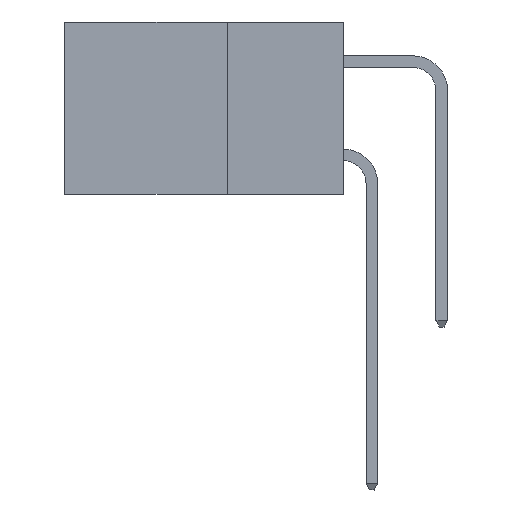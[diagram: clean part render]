
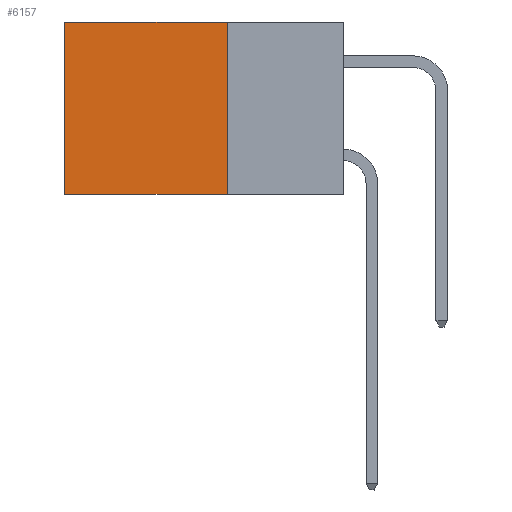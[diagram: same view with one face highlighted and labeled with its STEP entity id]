
A CAD part, left-side view. The second image highlights one B-rep face of the part: STEP entity #6157.
In plain terms, the highlighted planar face has unit normal (-1, 0, 0).
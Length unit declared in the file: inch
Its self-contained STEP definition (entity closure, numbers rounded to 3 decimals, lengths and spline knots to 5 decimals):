
#418 = LINE ( 'NONE', #6968, #10763 ) ;
#578 = DIRECTION ( 'NONE',  ( 1., 0., 0. ) ) ;
#1330 = EDGE_CURVE ( 'NONE', #8592, #1725, #4603, .T. ) ;
#1354 = ORIENTED_EDGE ( 'NONE', *, *, #11904, .T. ) ;
#1395 = EDGE_CURVE ( 'NONE', #2893, #11757, #418, .T. ) ;
#1702 = FACE_OUTER_BOUND ( 'NONE', #3119, .T. ) ;
#1725 = VERTEX_POINT ( 'NONE', #7755 ) ;
#2592 = DIRECTION ( 'NONE',  ( 0., 0., -1. ) ) ;
#2893 = VERTEX_POINT ( 'NONE', #11083 ) ;
#3119 = EDGE_LOOP ( 'NONE', ( #5556, #5331, #3422, #1354 ) ) ;
#3422 = ORIENTED_EDGE ( 'NONE', *, *, #1330, .F. ) ;
#3495 = DIRECTION ( 'NONE',  ( 0., 1., 0. ) ) ;
#4603 = LINE ( 'NONE', #7772, #11085 ) ;
#5016 = DIRECTION ( 'NONE',  ( 0., 0., -1. ) ) ;
#5331 = ORIENTED_EDGE ( 'NONE', *, *, #7487, .F. ) ;
#5556 = ORIENTED_EDGE ( 'NONE', *, *, #1395, .T. ) ;
#5565 = LINE ( 'NONE', #10313, #7311 ) ;
#5590 = CARTESIAN_POINT ( 'NONE',  ( 0.298, 0.6, -0.37 ) ) ;
#5743 = CARTESIAN_POINT ( 'NONE',  ( 0.298, 0.25, 0. ) ) ;
#6157 = ADVANCED_FACE ( 'NONE', ( #1702 ), #10578, .F. ) ;
#6539 = CARTESIAN_POINT ( 'NONE',  ( 0.298, 0.25, 0. ) ) ;
#6968 = CARTESIAN_POINT ( 'NONE',  ( 0.298, 0.6, 0. ) ) ;
#7311 = VECTOR ( 'NONE', #3495, 39.37008 ) ;
#7487 = EDGE_CURVE ( 'NONE', #1725, #11757, #5565, .T. ) ;
#7681 = VECTOR ( 'NONE', #10913, 39.37008 ) ;
#7755 = CARTESIAN_POINT ( 'NONE',  ( 0.298, 0.25, -0.37 ) ) ;
#7772 = CARTESIAN_POINT ( 'NONE',  ( 0.298, 0.25, 0. ) ) ;
#8116 = DIRECTION ( 'NONE',  ( 0., 0., -1. ) ) ;
#8324 = LINE ( 'NONE', #5743, #7681 ) ;
#8592 = VERTEX_POINT ( 'NONE', #10537 ) ;
#10313 = CARTESIAN_POINT ( 'NONE',  ( 0.298, 0.25, -0.37 ) ) ;
#10537 = CARTESIAN_POINT ( 'NONE',  ( 0.298, 0.25, 0. ) ) ;
#10578 = PLANE ( 'NONE',  #10631 ) ;
#10631 = AXIS2_PLACEMENT_3D ( 'NONE', #6539, #578, #2592 ) ;
#10763 = VECTOR ( 'NONE', #5016, 39.37008 ) ;
#10913 = DIRECTION ( 'NONE',  ( 0., 1., 0. ) ) ;
#11083 = CARTESIAN_POINT ( 'NONE',  ( 0.298, 0.6, 0. ) ) ;
#11085 = VECTOR ( 'NONE', #8116, 39.37008 ) ;
#11757 = VERTEX_POINT ( 'NONE', #5590 ) ;
#11904 = EDGE_CURVE ( 'NONE', #8592, #2893, #8324, .T. ) ;
